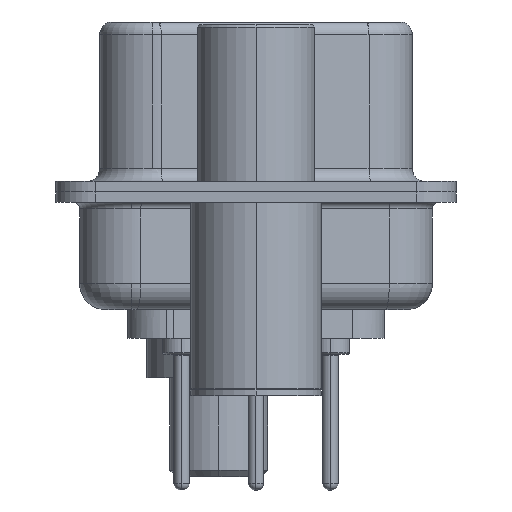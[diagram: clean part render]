
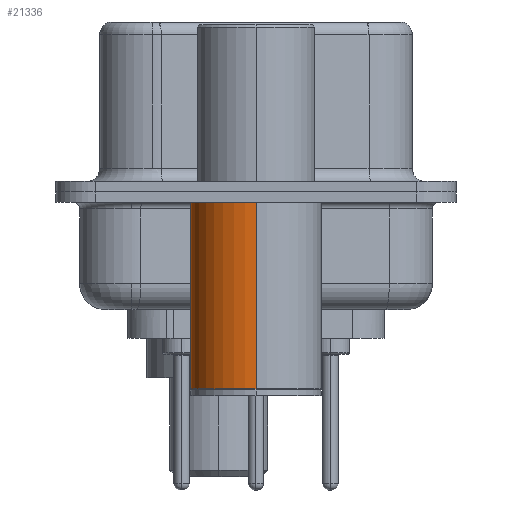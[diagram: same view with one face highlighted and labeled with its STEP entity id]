
A CAD part, left-side view. The second image highlights one B-rep face of the part: STEP entity #21336.
In plain terms, the highlighted cylindrical face has radius 2.5 mm (diameter 5 mm), a partial arc.
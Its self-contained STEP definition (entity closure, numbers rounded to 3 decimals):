
#509 = DIRECTION ( 'NONE',  ( 0., 0., 1. ) ) ;
#1025 = AXIS2_PLACEMENT_3D ( 'NONE', #27234, #509, #8033 ) ;
#2297 = CARTESIAN_POINT ( 'NONE',  ( 2.5, 0., -7.525 ) ) ;
#3837 = ORIENTED_EDGE ( 'NONE', *, *, #5180, .F. ) ;
#4111 = ORIENTED_EDGE ( 'NONE', *, *, #28819, .T. ) ;
#4391 = CARTESIAN_POINT ( 'NONE',  ( -2.5, 0., -7.525 ) ) ;
#5180 = EDGE_CURVE ( 'NONE', #29534, #20865, #18808, .T. ) ;
#5328 = VECTOR ( 'NONE', #8493, 1000. ) ;
#5495 = AXIS2_PLACEMENT_3D ( 'NONE', #20540, #26910, #27563 ) ;
#5813 = AXIS2_PLACEMENT_3D ( 'NONE', #10820, #27652, #13227 ) ;
#6017 = EDGE_CURVE ( 'NONE', #29534, #13169, #23242, .T. ) ;
#8033 = DIRECTION ( 'NONE',  ( 1., 0., 0. ) ) ;
#8493 = DIRECTION ( 'NONE',  ( 0., 0., 1. ) ) ;
#8532 = CARTESIAN_POINT ( 'NONE',  ( -2.5, 0., 0.581 ) ) ;
#8713 = EDGE_LOOP ( 'NONE', ( #13153, #4111, #15809, #3837 ) ) ;
#10820 = CARTESIAN_POINT ( 'NONE',  ( 0., 0., -0.4 ) ) ;
#10842 = CARTESIAN_POINT ( 'NONE',  ( 2.5, 0., 0.581 ) ) ;
#11088 = CARTESIAN_POINT ( 'NONE',  ( 2.5, 0., -0.4 ) ) ;
#12298 = LINE ( 'NONE', #8532, #30782 ) ;
#13153 = ORIENTED_EDGE ( 'NONE', *, *, #6017, .T. ) ;
#13169 = VERTEX_POINT ( 'NONE', #4391 ) ;
#13174 = CIRCLE ( 'NONE', #5813, 2.5 ) ;
#13227 = DIRECTION ( 'NONE',  ( 1., 0., 0. ) ) ;
#15809 = ORIENTED_EDGE ( 'NONE', *, *, #25747, .F. ) ;
#17876 = CYLINDRICAL_SURFACE ( 'NONE', #1025, 2.5 ) ;
#18808 = LINE ( 'NONE', #10842, #5328 ) ;
#20540 = CARTESIAN_POINT ( 'NONE',  ( 0., 0., -7.525 ) ) ;
#20865 = VERTEX_POINT ( 'NONE', #11088 ) ;
#20894 = FACE_OUTER_BOUND ( 'NONE', #8713, .T. ) ;
#21336 = ADVANCED_FACE ( 'NONE', ( #20894 ), #17876, .T. ) ;
#21955 = VERTEX_POINT ( 'NONE', #24826 ) ;
#23242 = CIRCLE ( 'NONE', #5495, 2.5 ) ;
#24826 = CARTESIAN_POINT ( 'NONE',  ( -2.5, 0., -0.4 ) ) ;
#25747 = EDGE_CURVE ( 'NONE', #20865, #21955, #13174, .T. ) ;
#26910 = DIRECTION ( 'NONE',  ( 0., 0., 1. ) ) ;
#27234 = CARTESIAN_POINT ( 'NONE',  ( 0., 0., 0.581 ) ) ;
#27563 = DIRECTION ( 'NONE',  ( 1., 0., 0. ) ) ;
#27652 = DIRECTION ( 'NONE',  ( 0., 0., 1. ) ) ;
#28819 = EDGE_CURVE ( 'NONE', #13169, #21955, #12298, .T. ) ;
#29534 = VERTEX_POINT ( 'NONE', #2297 ) ;
#30174 = DIRECTION ( 'NONE',  ( 0., 0., 1. ) ) ;
#30782 = VECTOR ( 'NONE', #30174, 1000. ) ;
